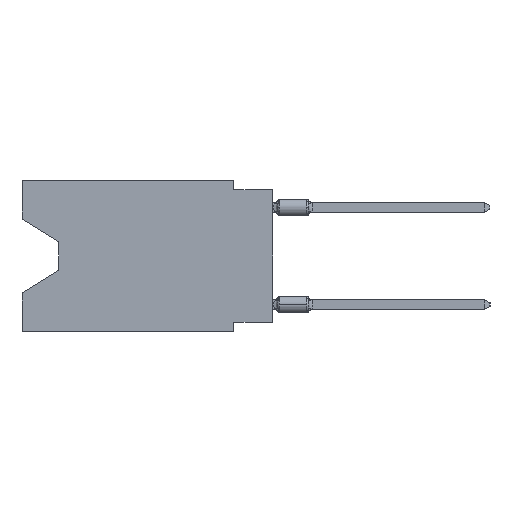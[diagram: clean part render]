
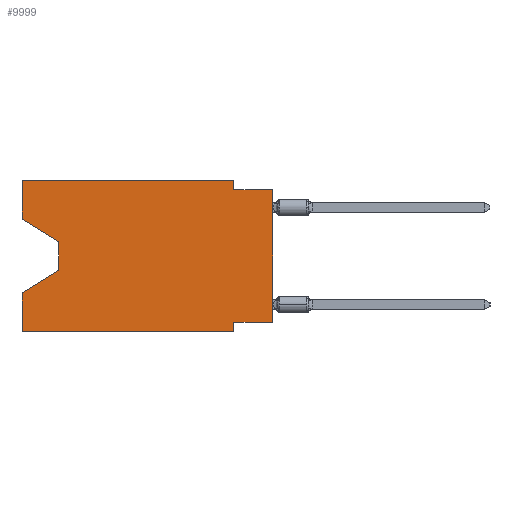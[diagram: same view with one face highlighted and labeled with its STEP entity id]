
A CAD part, left-side view. The second image highlights one B-rep face of the part: STEP entity #9999.
In plain terms, the highlighted planar face has unit normal (-1, 0, 0).
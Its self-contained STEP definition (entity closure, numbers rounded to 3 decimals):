
#261 = DIRECTION ( 'NONE',  ( 0., -1., 0. ) ) ;
#413 = CARTESIAN_POINT ( 'NONE',  ( 0., 2.54, -9.271 ) ) ;
#650 = LINE ( 'NONE', #18029, #11977 ) ;
#795 = VERTEX_POINT ( 'NONE', #22027 ) ;
#2038 = ORIENTED_EDGE ( 'NONE', *, *, #13340, .T. ) ;
#2655 = EDGE_CURVE ( 'NONE', #34834, #2798, #18664, .T. ) ;
#2798 = VERTEX_POINT ( 'NONE', #28344 ) ;
#4158 = CARTESIAN_POINT ( 'NONE',  ( 0., 16.383, 0. ) ) ;
#4251 = LINE ( 'NONE', #16022, #26783 ) ;
#4269 = VERTEX_POINT ( 'NONE', #33998 ) ;
#4323 = LINE ( 'NONE', #11063, #25386 ) ;
#4443 = CARTESIAN_POINT ( 'NONE',  ( 0., 16.383, -2.546 ) ) ;
#4789 = VERTEX_POINT ( 'NONE', #26220 ) ;
#5049 = EDGE_CURVE ( 'NONE', #11494, #34834, #14260, .T. ) ;
#5836 = VECTOR ( 'NONE', #22706, 1000. ) ;
#7393 = ORIENTED_EDGE ( 'NONE', *, *, #18869, .F. ) ;
#7596 = ORIENTED_EDGE ( 'NONE', *, *, #2655, .F. ) ;
#7703 = EDGE_CURVE ( 'NONE', #25027, #4789, #4251, .T. ) ;
#7806 = DIRECTION ( 'NONE',  ( 0., 0., 1. ) ) ;
#8275 = CARTESIAN_POINT ( 'NONE',  ( 0., 0., -9.271 ) ) ;
#8752 = EDGE_CURVE ( 'NONE', #30735, #24285, #34015, .T. ) ;
#9999 = ADVANCED_FACE ( 'NONE', ( #15786 ), #20825, .F. ) ;
#10115 = CARTESIAN_POINT ( 'NONE',  ( 0., 16.383, 0. ) ) ;
#10444 = EDGE_CURVE ( 'NONE', #795, #25620, #21928, .T. ) ;
#10687 = DIRECTION ( 'NONE',  ( 0., 0., 1. ) ) ;
#10797 = VECTOR ( 'NONE', #27233, 1000. ) ;
#10859 = ORIENTED_EDGE ( 'NONE', *, *, #13828, .F. ) ;
#11063 = CARTESIAN_POINT ( 'NONE',  ( 0., 0., 0. ) ) ;
#11494 = VERTEX_POINT ( 'NONE', #25441 ) ;
#11977 = VECTOR ( 'NONE', #261, 1000. ) ;
#12983 = VERTEX_POINT ( 'NONE', #17108 ) ;
#13132 = VECTOR ( 'NONE', #25782, 1000. ) ;
#13340 = EDGE_CURVE ( 'NONE', #33198, #25620, #13978, .T. ) ;
#13828 = EDGE_CURVE ( 'NONE', #4789, #4269, #34744, .T. ) ;
#13885 = DIRECTION ( 'NONE',  ( 0., -1., 0. ) ) ;
#13978 = LINE ( 'NONE', #23576, #13132 ) ;
#14079 = DIRECTION ( 'NONE',  ( 0., 1., 0. ) ) ;
#14260 = LINE ( 'NONE', #8275, #18045 ) ;
#14660 = ORIENTED_EDGE ( 'NONE', *, *, #5049, .F. ) ;
#15414 = CARTESIAN_POINT ( 'NONE',  ( 0., 16.383, -9.906 ) ) ;
#15559 = ORIENTED_EDGE ( 'NONE', *, *, #19410, .T. ) ;
#15786 = FACE_OUTER_BOUND ( 'NONE', #20024, .T. ) ;
#16022 = CARTESIAN_POINT ( 'NONE',  ( 0., 2.54, 0. ) ) ;
#16104 = AXIS2_PLACEMENT_3D ( 'NONE', #17918, #36101, #29726 ) ;
#16338 = CARTESIAN_POINT ( 'NONE',  ( 0., 13.97, -5.893 ) ) ;
#17108 = CARTESIAN_POINT ( 'NONE',  ( 0., 16.383, 0. ) ) ;
#17409 = EDGE_CURVE ( 'NONE', #24285, #33198, #28136, .T. ) ;
#17918 = CARTESIAN_POINT ( 'NONE',  ( 0., 16.383, 0. ) ) ;
#18029 = CARTESIAN_POINT ( 'NONE',  ( 0., 16.383, 0. ) ) ;
#18045 = VECTOR ( 'NONE', #14079, 1000. ) ;
#18664 = LINE ( 'NONE', #36645, #30670 ) ;
#18869 = EDGE_CURVE ( 'NONE', #12983, #25027, #650, .T. ) ;
#19234 = ORIENTED_EDGE ( 'NONE', *, *, #17409, .T. ) ;
#19400 = VECTOR ( 'NONE', #30734, 1000. ) ;
#19410 = EDGE_CURVE ( 'NONE', #795, #2798, #30130, .T. ) ;
#19423 = CARTESIAN_POINT ( 'NONE',  ( 0., 13.97, -4.013 ) ) ;
#20024 = EDGE_LOOP ( 'NONE', ( #23398, #19234, #2038, #27714, #15559, #7596, #14660, #22602, #10859, #23233, #7393, #20409 ) ) ;
#20409 = ORIENTED_EDGE ( 'NONE', *, *, #37493, .F. ) ;
#20432 = CARTESIAN_POINT ( 'NONE',  ( 0., 0., -0.635 ) ) ;
#20825 = PLANE ( 'NONE',  #16104 ) ;
#21928 = LINE ( 'NONE', #4158, #28161 ) ;
#22027 = CARTESIAN_POINT ( 'NONE',  ( 0., 16.383, -9.906 ) ) ;
#22602 = ORIENTED_EDGE ( 'NONE', *, *, #33637, .T. ) ;
#22706 = DIRECTION ( 'NONE',  ( 0., 0., -1. ) ) ;
#23233 = ORIENTED_EDGE ( 'NONE', *, *, #7703, .F. ) ;
#23398 = ORIENTED_EDGE ( 'NONE', *, *, #8752, .T. ) ;
#23576 = CARTESIAN_POINT ( 'NONE',  ( 0., 13.97, -5.893 ) ) ;
#24285 = VERTEX_POINT ( 'NONE', #24661 ) ;
#24661 = CARTESIAN_POINT ( 'NONE',  ( 0., 13.97, -4.013 ) ) ;
#24871 = VECTOR ( 'NONE', #13885, 1000. ) ;
#25013 = DIRECTION ( 'NONE',  ( 0., 0., 1. ) ) ;
#25027 = VERTEX_POINT ( 'NONE', #33263 ) ;
#25386 = VECTOR ( 'NONE', #25013, 1000. ) ;
#25441 = CARTESIAN_POINT ( 'NONE',  ( 0., 0., -9.271 ) ) ;
#25589 = LINE ( 'NONE', #10115, #35179 ) ;
#25620 = VERTEX_POINT ( 'NONE', #35295 ) ;
#25782 = DIRECTION ( 'NONE',  ( 0., 0.855, -0.519 ) ) ;
#26217 = CARTESIAN_POINT ( 'NONE',  ( 0., 16.383, -2.546 ) ) ;
#26220 = CARTESIAN_POINT ( 'NONE',  ( 0., 2.54, -0.635 ) ) ;
#26783 = VECTOR ( 'NONE', #27832, 1000. ) ;
#27193 = DIRECTION ( 'NONE',  ( 0., 0., -1. ) ) ;
#27233 = DIRECTION ( 'NONE',  ( 0., -1., 0. ) ) ;
#27714 = ORIENTED_EDGE ( 'NONE', *, *, #10444, .F. ) ;
#27832 = DIRECTION ( 'NONE',  ( 0., 0., -1. ) ) ;
#28136 = LINE ( 'NONE', #19423, #5836 ) ;
#28161 = VECTOR ( 'NONE', #7806, 1000. ) ;
#28344 = CARTESIAN_POINT ( 'NONE',  ( 0., 2.54, -9.906 ) ) ;
#29726 = DIRECTION ( 'NONE',  ( 0., 0., -1. ) ) ;
#30130 = LINE ( 'NONE', #15414, #10797 ) ;
#30670 = VECTOR ( 'NONE', #27193, 1000. ) ;
#30734 = DIRECTION ( 'NONE',  ( 0., -0.855, -0.519 ) ) ;
#30735 = VERTEX_POINT ( 'NONE', #26217 ) ;
#33198 = VERTEX_POINT ( 'NONE', #16338 ) ;
#33263 = CARTESIAN_POINT ( 'NONE',  ( 0., 2.54, 0. ) ) ;
#33637 = EDGE_CURVE ( 'NONE', #11494, #4269, #4323, .T. ) ;
#33998 = CARTESIAN_POINT ( 'NONE',  ( 0., 0., -0.635 ) ) ;
#34015 = LINE ( 'NONE', #4443, #19400 ) ;
#34744 = LINE ( 'NONE', #20432, #24871 ) ;
#34834 = VERTEX_POINT ( 'NONE', #413 ) ;
#35179 = VECTOR ( 'NONE', #10687, 1000. ) ;
#35295 = CARTESIAN_POINT ( 'NONE',  ( 0., 16.383, -7.36 ) ) ;
#36101 = DIRECTION ( 'NONE',  ( 1., 0., 0. ) ) ;
#36645 = CARTESIAN_POINT ( 'NONE',  ( 0., 2.54, -9.906 ) ) ;
#37493 = EDGE_CURVE ( 'NONE', #30735, #12983, #25589, .T. ) ;
